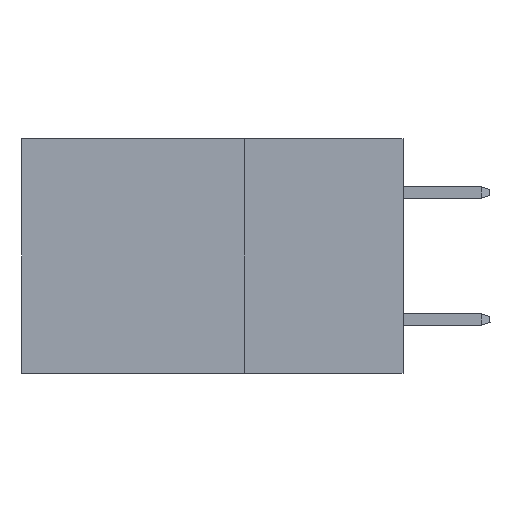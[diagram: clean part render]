
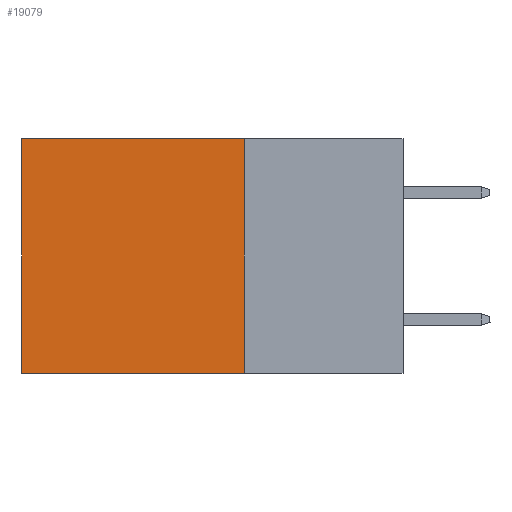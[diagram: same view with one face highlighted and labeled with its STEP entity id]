
A CAD part, left-side view. The second image highlights one B-rep face of the part: STEP entity #19079.
In plain terms, the highlighted planar face has unit normal (-1, 0, 0).
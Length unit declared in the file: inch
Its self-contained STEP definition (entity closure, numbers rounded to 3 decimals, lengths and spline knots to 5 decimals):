
#407 = VERTEX_POINT ( 'NONE', #13410 ) ;
#869 = AXIS2_PLACEMENT_3D ( 'NONE', #10914, #7405, #7281 ) ;
#948 = EDGE_CURVE ( 'NONE', #12089, #10278, #3116, .T. ) ;
#1231 = DIRECTION ( 'NONE',  ( 0., 0., -1. ) ) ;
#1843 = LINE ( 'NONE', #11411, #19842 ) ;
#2688 = VECTOR ( 'NONE', #1231, 39.37008 ) ;
#2830 = ORIENTED_EDGE ( 'NONE', *, *, #13471, .T. ) ;
#3116 = LINE ( 'NONE', #8818, #2688 ) ;
#3380 = VERTEX_POINT ( 'NONE', #12989 ) ;
#4882 = ORIENTED_EDGE ( 'NONE', *, *, #7879, .F. ) ;
#6116 = ORIENTED_EDGE ( 'NONE', *, *, #11793, .T. ) ;
#6342 = LINE ( 'NONE', #20283, #11824 ) ;
#7281 = DIRECTION ( 'NONE',  ( 0., 0., -1. ) ) ;
#7289 = DIRECTION ( 'NONE',  ( 0., 0., -1. ) ) ;
#7405 = DIRECTION ( 'NONE',  ( 1., 0., 0. ) ) ;
#7879 = EDGE_CURVE ( 'NONE', #10278, #407, #6342, .T. ) ;
#8818 = CARTESIAN_POINT ( 'NONE',  ( 0.2875, 0.25, 0. ) ) ;
#9704 = CARTESIAN_POINT ( 'NONE',  ( 0.2875, 0.25, 0. ) ) ;
#10278 = VERTEX_POINT ( 'NONE', #10413 ) ;
#10413 = CARTESIAN_POINT ( 'NONE',  ( 0.2875, 0.25, -0.37 ) ) ;
#10914 = CARTESIAN_POINT ( 'NONE',  ( 0.2875, 0.25, 0. ) ) ;
#11411 = CARTESIAN_POINT ( 'NONE',  ( 0.2875, 0.6, 0. ) ) ;
#11793 = EDGE_CURVE ( 'NONE', #3380, #407, #1843, .T. ) ;
#11824 = VECTOR ( 'NONE', #18434, 39.37008 ) ;
#12089 = VERTEX_POINT ( 'NONE', #12495 ) ;
#12495 = CARTESIAN_POINT ( 'NONE',  ( 0.2875, 0.25, 0. ) ) ;
#12646 = PLANE ( 'NONE',  #869 ) ;
#12989 = CARTESIAN_POINT ( 'NONE',  ( 0.2875, 0.6, 0. ) ) ;
#13410 = CARTESIAN_POINT ( 'NONE',  ( 0.2875, 0.6, -0.37 ) ) ;
#13471 = EDGE_CURVE ( 'NONE', #12089, #3380, #21390, .T. ) ;
#13805 = DIRECTION ( 'NONE',  ( 0., 1., 0. ) ) ;
#14520 = FACE_OUTER_BOUND ( 'NONE', #23387, .T. ) ;
#18318 = VECTOR ( 'NONE', #13805, 39.37008 ) ;
#18434 = DIRECTION ( 'NONE',  ( 0., 1., 0. ) ) ;
#19079 = ADVANCED_FACE ( 'NONE', ( #14520 ), #12646, .F. ) ;
#19842 = VECTOR ( 'NONE', #7289, 39.37008 ) ;
#20239 = ORIENTED_EDGE ( 'NONE', *, *, #948, .F. ) ;
#20283 = CARTESIAN_POINT ( 'NONE',  ( 0.2875, 0.25, -0.37 ) ) ;
#21390 = LINE ( 'NONE', #9704, #18318 ) ;
#23387 = EDGE_LOOP ( 'NONE', ( #6116, #4882, #20239, #2830 ) ) ;
